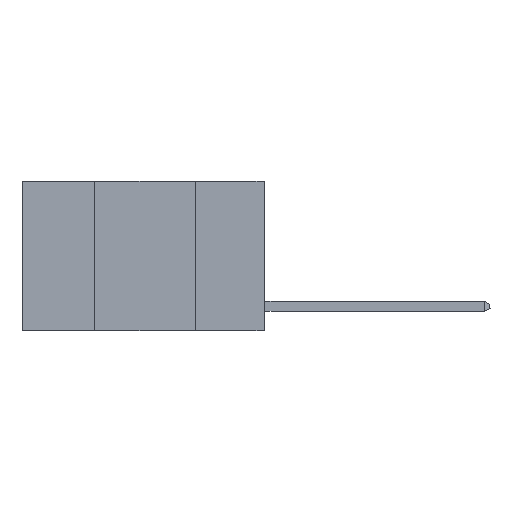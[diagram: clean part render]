
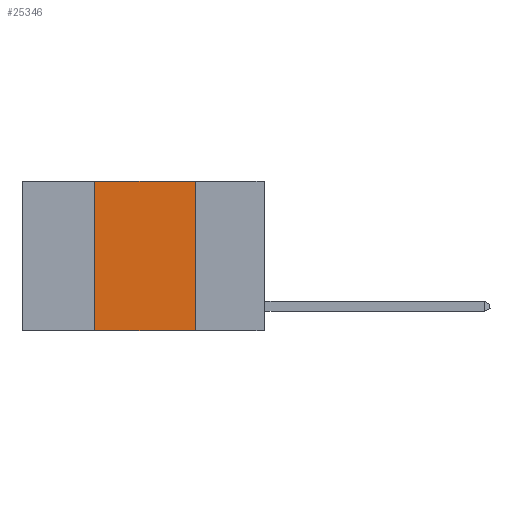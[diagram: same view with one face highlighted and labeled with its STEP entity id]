
A CAD part, left-side view. The second image highlights one B-rep face of the part: STEP entity #25346.
In plain terms, the highlighted planar face has unit normal (-1, 0, 0).
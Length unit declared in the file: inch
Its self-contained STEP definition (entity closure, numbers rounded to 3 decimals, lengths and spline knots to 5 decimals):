
#629 = CARTESIAN_POINT ( 'NONE',  ( 0., 0.42, 0. ) ) ;
#922 = CARTESIAN_POINT ( 'NONE',  ( 0., 0.17, -0.37 ) ) ;
#926 = VERTEX_POINT ( 'NONE', #922 ) ;
#943 = CARTESIAN_POINT ( 'NONE',  ( 0., 0.17, 0. ) ) ;
#1657 = DIRECTION ( 'NONE',  ( 0., -1., 0. ) ) ;
#2161 = VERTEX_POINT ( 'NONE', #943 ) ;
#2733 = DIRECTION ( 'NONE',  ( 0., 0., 1. ) ) ;
#2900 = CARTESIAN_POINT ( 'NONE',  ( 0., 0.6, -0.37 ) ) ;
#3172 = CARTESIAN_POINT ( 'NONE',  ( 0., 0.17, 0. ) ) ;
#4018 = LINE ( 'NONE', #3172, #19465 ) ;
#4718 = PLANE ( 'NONE',  #21489 ) ;
#5817 = CARTESIAN_POINT ( 'NONE',  ( 0., 0.6, 0. ) ) ;
#6400 = VERTEX_POINT ( 'NONE', #23896 ) ;
#6772 = DIRECTION ( 'NONE',  ( 1., 0., 0. ) ) ;
#6912 = EDGE_CURVE ( 'NONE', #17529, #2161, #22283, .T. ) ;
#6996 = CARTESIAN_POINT ( 'NONE',  ( 0., 0.42, 0. ) ) ;
#7220 = EDGE_CURVE ( 'NONE', #6400, #17529, #18852, .T. ) ;
#8502 = ORIENTED_EDGE ( 'NONE', *, *, #7220, .F. ) ;
#8823 = VECTOR ( 'NONE', #2733, 39.37008 ) ;
#9072 = DIRECTION ( 'NONE',  ( 0., -1., 0. ) ) ;
#11491 = VECTOR ( 'NONE', #9072, 39.37008 ) ;
#12707 = ORIENTED_EDGE ( 'NONE', *, *, #6912, .F. ) ;
#13029 = ORIENTED_EDGE ( 'NONE', *, *, #16964, .F. ) ;
#16831 = LINE ( 'NONE', #2900, #11491 ) ;
#16964 = EDGE_CURVE ( 'NONE', #2161, #926, #4018, .T. ) ;
#17529 = VERTEX_POINT ( 'NONE', #6996 ) ;
#18803 = CARTESIAN_POINT ( 'NONE',  ( 0., 0.6, 0. ) ) ;
#18852 = LINE ( 'NONE', #629, #8823 ) ;
#19318 = DIRECTION ( 'NONE',  ( 0., 0., -1. ) ) ;
#19465 = VECTOR ( 'NONE', #19318, 39.37008 ) ;
#19628 = EDGE_CURVE ( 'NONE', #6400, #926, #16831, .T. ) ;
#19975 = ORIENTED_EDGE ( 'NONE', *, *, #19628, .T. ) ;
#20800 = DIRECTION ( 'NONE',  ( 0., 0., -1. ) ) ;
#21489 = AXIS2_PLACEMENT_3D ( 'NONE', #18803, #6772, #20800 ) ;
#21651 = VECTOR ( 'NONE', #1657, 39.37008 ) ;
#22283 = LINE ( 'NONE', #5817, #21651 ) ;
#22663 = FACE_OUTER_BOUND ( 'NONE', #25271, .T. ) ;
#23896 = CARTESIAN_POINT ( 'NONE',  ( 0., 0.42, -0.37 ) ) ;
#25271 = EDGE_LOOP ( 'NONE', ( #13029, #12707, #8502, #19975 ) ) ;
#25346 = ADVANCED_FACE ( 'NONE', ( #22663 ), #4718, .F. ) ;
